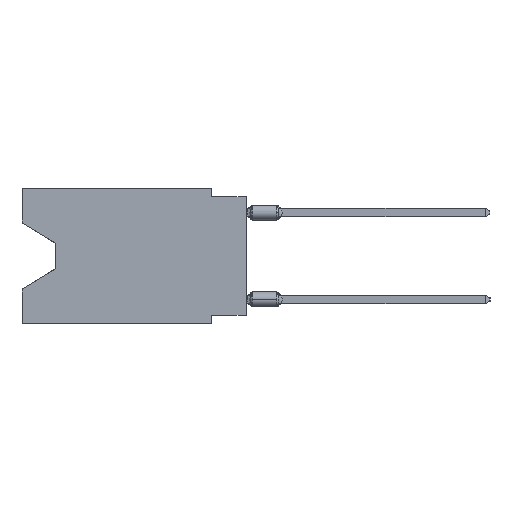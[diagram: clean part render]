
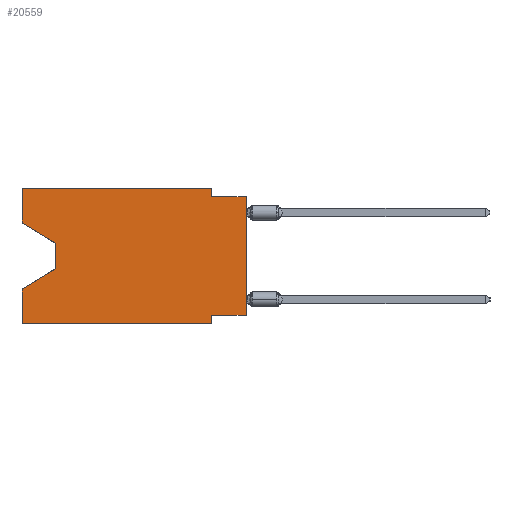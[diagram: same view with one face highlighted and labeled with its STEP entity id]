
A CAD part, left-side view. The second image highlights one B-rep face of the part: STEP entity #20559.
In plain terms, the highlighted planar face has unit normal (-1, 0, 0).
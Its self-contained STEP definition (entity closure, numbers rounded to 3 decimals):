
#177 = CARTESIAN_POINT ( 'NONE',  ( 0., 2.54, 0. ) ) ;
#1476 = ORIENTED_EDGE ( 'NONE', *, *, #19808, .F. ) ;
#1548 = EDGE_CURVE ( 'NONE', #23545, #31161, #3748, .T. ) ;
#2040 = VERTEX_POINT ( 'NONE', #40905 ) ;
#2090 = EDGE_CURVE ( 'NONE', #13028, #3908, #8694, .T. ) ;
#3037 = CARTESIAN_POINT ( 'NONE',  ( 0., 2.54, -0.635 ) ) ;
#3409 = CARTESIAN_POINT ( 'NONE',  ( 0., 16.383, -7.36 ) ) ;
#3748 = LINE ( 'NONE', #3974, #12666 ) ;
#3908 = VERTEX_POINT ( 'NONE', #3409 ) ;
#3974 = CARTESIAN_POINT ( 'NONE',  ( 0., 16.383, -2.546 ) ) ;
#4582 = ORIENTED_EDGE ( 'NONE', *, *, #21024, .T. ) ;
#4667 = DIRECTION ( 'NONE',  ( 1., 0., 0. ) ) ;
#4725 = DIRECTION ( 'NONE',  ( 0., -1., 0. ) ) ;
#5542 = DIRECTION ( 'NONE',  ( 0., 0., 1. ) ) ;
#6114 = CARTESIAN_POINT ( 'NONE',  ( 0., 16.383, -2.546 ) ) ;
#6684 = LINE ( 'NONE', #23608, #44933 ) ;
#6887 = CARTESIAN_POINT ( 'NONE',  ( 0., 13.97, -4.013 ) ) ;
#7372 = LINE ( 'NONE', #14228, #9573 ) ;
#8141 = VECTOR ( 'NONE', #27222, 1000. ) ;
#8273 = DIRECTION ( 'NONE',  ( 0., -1., 0. ) ) ;
#8609 = CARTESIAN_POINT ( 'NONE',  ( 0., 16.383, 0. ) ) ;
#8663 = ORIENTED_EDGE ( 'NONE', *, *, #1548, .T. ) ;
#8694 = LINE ( 'NONE', #12962, #19156 ) ;
#9573 = VECTOR ( 'NONE', #31415, 1000. ) ;
#9655 = CARTESIAN_POINT ( 'NONE',  ( 0., 0., 0. ) ) ;
#9987 = CARTESIAN_POINT ( 'NONE',  ( 0., 2.54, -9.271 ) ) ;
#10919 = ORIENTED_EDGE ( 'NONE', *, *, #2090, .T. ) ;
#11590 = LINE ( 'NONE', #8609, #19811 ) ;
#12666 = VECTOR ( 'NONE', #35990, 1000. ) ;
#12673 = VERTEX_POINT ( 'NONE', #19954 ) ;
#12962 = CARTESIAN_POINT ( 'NONE',  ( 0., 13.97, -5.893 ) ) ;
#13028 = VERTEX_POINT ( 'NONE', #16704 ) ;
#13381 = ORIENTED_EDGE ( 'NONE', *, *, #35805, .F. ) ;
#13511 = EDGE_LOOP ( 'NONE', ( #8663, #17473, #10919, #39705, #4582, #1476, #30973, #17970, #14926, #23401, #32348, #13381 ) ) ;
#14228 = CARTESIAN_POINT ( 'NONE',  ( 0., 0., -9.271 ) ) ;
#14283 = AXIS2_PLACEMENT_3D ( 'NONE', #21589, #4667, #36470 ) ;
#14926 = ORIENTED_EDGE ( 'NONE', *, *, #29556, .F. ) ;
#15436 = VECTOR ( 'NONE', #43995, 1000. ) ;
#15791 = EDGE_CURVE ( 'NONE', #2040, #31434, #7372, .T. ) ;
#15984 = VECTOR ( 'NONE', #36318, 1000. ) ;
#15989 = VECTOR ( 'NONE', #17223, 1000. ) ;
#16091 = EDGE_CURVE ( 'NONE', #39767, #33400, #23332, .T. ) ;
#16230 = CARTESIAN_POINT ( 'NONE',  ( 0., 2.54, 0. ) ) ;
#16704 = CARTESIAN_POINT ( 'NONE',  ( 0., 13.97, -5.893 ) ) ;
#16852 = EDGE_CURVE ( 'NONE', #21454, #39767, #11590, .T. ) ;
#17001 = VERTEX_POINT ( 'NONE', #26214 ) ;
#17223 = DIRECTION ( 'NONE',  ( 0., 0., 1. ) ) ;
#17473 = ORIENTED_EDGE ( 'NONE', *, *, #18381, .T. ) ;
#17970 = ORIENTED_EDGE ( 'NONE', *, *, #18385, .T. ) ;
#18381 = EDGE_CURVE ( 'NONE', #31161, #13028, #36895, .T. ) ;
#18385 = EDGE_CURVE ( 'NONE', #2040, #17001, #37580, .T. ) ;
#19156 = VECTOR ( 'NONE', #36160, 1000. ) ;
#19175 = VECTOR ( 'NONE', #38725, 1000. ) ;
#19808 = EDGE_CURVE ( 'NONE', #31434, #12673, #42172, .T. ) ;
#19811 = VECTOR ( 'NONE', #4725, 1000. ) ;
#19954 = CARTESIAN_POINT ( 'NONE',  ( 0., 2.54, -9.906 ) ) ;
#20559 = ADVANCED_FACE ( 'NONE', ( #29154 ), #22038, .F. ) ;
#20601 = VERTEX_POINT ( 'NONE', #22492 ) ;
#21024 = EDGE_CURVE ( 'NONE', #20601, #12673, #21528, .T. ) ;
#21454 = VERTEX_POINT ( 'NONE', #42123 ) ;
#21528 = LINE ( 'NONE', #42399, #39182 ) ;
#21589 = CARTESIAN_POINT ( 'NONE',  ( 0., 16.383, 0. ) ) ;
#22038 = PLANE ( 'NONE',  #14283 ) ;
#22492 = CARTESIAN_POINT ( 'NONE',  ( 0., 16.383, -9.906 ) ) ;
#23239 = LINE ( 'NONE', #36540, #15984 ) ;
#23332 = LINE ( 'NONE', #16230, #8141 ) ;
#23374 = CARTESIAN_POINT ( 'NONE',  ( 0., 13.97, -4.013 ) ) ;
#23401 = ORIENTED_EDGE ( 'NONE', *, *, #16091, .F. ) ;
#23545 = VERTEX_POINT ( 'NONE', #6114 ) ;
#23608 = CARTESIAN_POINT ( 'NONE',  ( 0., 0., -0.635 ) ) ;
#24748 = CARTESIAN_POINT ( 'NONE',  ( 0., 2.54, -9.906 ) ) ;
#25666 = VECTOR ( 'NONE', #5542, 1000. ) ;
#26214 = CARTESIAN_POINT ( 'NONE',  ( 0., 0., -0.635 ) ) ;
#27222 = DIRECTION ( 'NONE',  ( 0., 0., -1. ) ) ;
#27300 = CARTESIAN_POINT ( 'NONE',  ( 0., 16.383, 0. ) ) ;
#29154 = FACE_OUTER_BOUND ( 'NONE', #13511, .T. ) ;
#29556 = EDGE_CURVE ( 'NONE', #33400, #17001, #6684, .T. ) ;
#30973 = ORIENTED_EDGE ( 'NONE', *, *, #15791, .F. ) ;
#31161 = VERTEX_POINT ( 'NONE', #6887 ) ;
#31415 = DIRECTION ( 'NONE',  ( 0., 1., 0. ) ) ;
#31434 = VERTEX_POINT ( 'NONE', #9987 ) ;
#32348 = ORIENTED_EDGE ( 'NONE', *, *, #16852, .F. ) ;
#33400 = VERTEX_POINT ( 'NONE', #3037 ) ;
#34605 = DIRECTION ( 'NONE',  ( 0., -1., 0. ) ) ;
#35805 = EDGE_CURVE ( 'NONE', #23545, #21454, #23239, .T. ) ;
#35990 = DIRECTION ( 'NONE',  ( 0., -0.855, -0.519 ) ) ;
#36160 = DIRECTION ( 'NONE',  ( 0., 0.855, -0.519 ) ) ;
#36318 = DIRECTION ( 'NONE',  ( 0., 0., 1. ) ) ;
#36470 = DIRECTION ( 'NONE',  ( 0., 0., -1. ) ) ;
#36540 = CARTESIAN_POINT ( 'NONE',  ( 0., 16.383, 0. ) ) ;
#36895 = LINE ( 'NONE', #23374, #15436 ) ;
#37580 = LINE ( 'NONE', #9655, #25666 ) ;
#38725 = DIRECTION ( 'NONE',  ( 0., 0., -1. ) ) ;
#39182 = VECTOR ( 'NONE', #8273, 1000. ) ;
#39705 = ORIENTED_EDGE ( 'NONE', *, *, #45018, .F. ) ;
#39767 = VERTEX_POINT ( 'NONE', #177 ) ;
#40905 = CARTESIAN_POINT ( 'NONE',  ( 0., 0., -9.271 ) ) ;
#41956 = LINE ( 'NONE', #27300, #15989 ) ;
#42123 = CARTESIAN_POINT ( 'NONE',  ( 0., 16.383, 0. ) ) ;
#42172 = LINE ( 'NONE', #24748, #19175 ) ;
#42399 = CARTESIAN_POINT ( 'NONE',  ( 0., 16.383, -9.906 ) ) ;
#43995 = DIRECTION ( 'NONE',  ( 0., 0., -1. ) ) ;
#44933 = VECTOR ( 'NONE', #34605, 1000. ) ;
#45018 = EDGE_CURVE ( 'NONE', #20601, #3908, #41956, .T. ) ;
